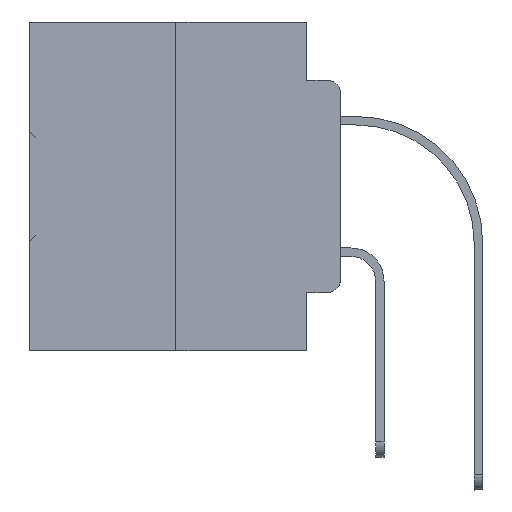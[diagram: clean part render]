
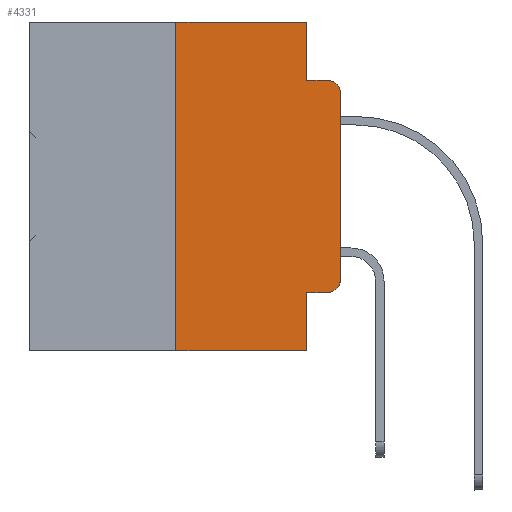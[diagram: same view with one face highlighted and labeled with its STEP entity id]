
A CAD part, left-side view. The second image highlights one B-rep face of the part: STEP entity #4331.
In plain terms, the highlighted planar face has unit normal (-1, 0, 0).
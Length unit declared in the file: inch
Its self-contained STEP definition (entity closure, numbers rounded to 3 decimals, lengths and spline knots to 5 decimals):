
#71 = VERTEX_POINT ( 'NONE', #11386 ) ;
#820 = VECTOR ( 'NONE', #32199, 39.37008 ) ;
#951 = VERTEX_POINT ( 'NONE', #14793 ) ;
#1387 = ORIENTED_EDGE ( 'NONE', *, *, #4646, .T. ) ;
#2530 = CARTESIAN_POINT ( 'NONE',  ( 0., 0.02, -0.1085 ) ) ;
#2739 = CARTESIAN_POINT ( 'NONE',  ( 0., 0.25, 0. ) ) ;
#3098 = VECTOR ( 'NONE', #36138, 39.37008 ) ;
#3519 = AXIS2_PLACEMENT_3D ( 'NONE', #2530, #40285, #39898 ) ;
#3543 = ORIENTED_EDGE ( 'NONE', *, *, #11074, .T. ) ;
#3774 = CARTESIAN_POINT ( 'NONE',  ( 0., 0.25, 0. ) ) ;
#3966 = EDGE_CURVE ( 'NONE', #38152, #21400, #7041, .T. ) ;
#4331 = ADVANCED_FACE ( 'NONE', ( #37162 ), #15233, .F. ) ;
#4646 = EDGE_CURVE ( 'NONE', #7658, #6983, #12684, .T. ) ;
#6547 = ORIENTED_EDGE ( 'NONE', *, *, #21950, .T. ) ;
#6983 = VERTEX_POINT ( 'NONE', #37576 ) ;
#7041 = LINE ( 'NONE', #25828, #21017 ) ;
#7658 = VERTEX_POINT ( 'NONE', #33580 ) ;
#7666 = ORIENTED_EDGE ( 'NONE', *, *, #16347, .F. ) ;
#10382 = ORIENTED_EDGE ( 'NONE', *, *, #17282, .T. ) ;
#11074 = EDGE_CURVE ( 'NONE', #951, #21400, #35186, .T. ) ;
#11386 = CARTESIAN_POINT ( 'NONE',  ( 0., 0.051, 0. ) ) ;
#11757 = CARTESIAN_POINT ( 'NONE',  ( 0., 0.02, -0.0885 ) ) ;
#12130 = VECTOR ( 'NONE', #33326, 39.37008 ) ;
#12591 = VERTEX_POINT ( 'NONE', #33820 ) ;
#12684 = CIRCLE ( 'NONE', #19306, 0.02 ) ;
#13681 = EDGE_CURVE ( 'NONE', #12591, #31669, #24660, .T. ) ;
#13884 = LINE ( 'NONE', #26511, #12130 ) ;
#14793 = CARTESIAN_POINT ( 'NONE',  ( 0., 0., -0.1085 ) ) ;
#14946 = CARTESIAN_POINT ( 'NONE',  ( 0., 0.02, -0.3915 ) ) ;
#15233 = PLANE ( 'NONE',  #28963 ) ;
#16347 = EDGE_CURVE ( 'NONE', #71, #38152, #23553, .T. ) ;
#16421 = CARTESIAN_POINT ( 'NONE',  ( 0., 0.051, -0.5 ) ) ;
#17098 = LINE ( 'NONE', #25800, #820 ) ;
#17282 = EDGE_CURVE ( 'NONE', #6983, #951, #18667, .T. ) ;
#17742 = CARTESIAN_POINT ( 'NONE',  ( 0., 0.051, 0. ) ) ;
#18364 = DIRECTION ( 'NONE',  ( 1., 0., 0. ) ) ;
#18667 = LINE ( 'NONE', #31278, #34180 ) ;
#19306 = AXIS2_PLACEMENT_3D ( 'NONE', #14946, #27579, #31486 ) ;
#19675 = EDGE_LOOP ( 'NONE', ( #10382, #3543, #33241, #7666, #37746, #26493, #24767, #35890, #6547, #1387 ) ) ;
#20393 = CARTESIAN_POINT ( 'NONE',  ( 0., 0.051, 0. ) ) ;
#21017 = VECTOR ( 'NONE', #35334, 39.37008 ) ;
#21400 = VERTEX_POINT ( 'NONE', #11757 ) ;
#21603 = EDGE_CURVE ( 'NONE', #12591, #27173, #17098, .T. ) ;
#21883 = VECTOR ( 'NONE', #37523, 39.37008 ) ;
#21950 = EDGE_CURVE ( 'NONE', #32676, #7658, #37342, .T. ) ;
#23521 = LINE ( 'NONE', #20393, #21883 ) ;
#23553 = LINE ( 'NONE', #17742, #3098 ) ;
#24660 = LINE ( 'NONE', #2739, #35151 ) ;
#24767 = ORIENTED_EDGE ( 'NONE', *, *, #21603, .T. ) ;
#24891 = CARTESIAN_POINT ( 'NONE',  ( 0., 0.051, -0.0885 ) ) ;
#25800 = CARTESIAN_POINT ( 'NONE',  ( 0., 0.473, -0.5 ) ) ;
#25828 = CARTESIAN_POINT ( 'NONE',  ( 0., 0.051, -0.0885 ) ) ;
#26493 = ORIENTED_EDGE ( 'NONE', *, *, #13681, .F. ) ;
#26511 = CARTESIAN_POINT ( 'NONE',  ( 0., 0.473, 0. ) ) ;
#26810 = CARTESIAN_POINT ( 'NONE',  ( 0., 0.051, -0.4115 ) ) ;
#26950 = EDGE_CURVE ( 'NONE', #32676, #27173, #23521, .T. ) ;
#27173 = VERTEX_POINT ( 'NONE', #16421 ) ;
#27264 = CARTESIAN_POINT ( 'NONE',  ( 0., 0.473, 0. ) ) ;
#27377 = DIRECTION ( 'NONE',  ( 0., 0., 1. ) ) ;
#27579 = DIRECTION ( 'NONE',  ( -1., 0., 0. ) ) ;
#28255 = DIRECTION ( 'NONE',  ( 0., -1., 0. ) ) ;
#28668 = EDGE_CURVE ( 'NONE', #31669, #71, #13884, .T. ) ;
#28963 = AXIS2_PLACEMENT_3D ( 'NONE', #27264, #18364, #33637 ) ;
#30565 = VECTOR ( 'NONE', #28255, 39.37008 ) ;
#31278 = CARTESIAN_POINT ( 'NONE',  ( 0., 0., 0. ) ) ;
#31486 = DIRECTION ( 'NONE',  ( 0., 0., -1. ) ) ;
#31669 = VERTEX_POINT ( 'NONE', #3774 ) ;
#31735 = CARTESIAN_POINT ( 'NONE',  ( 0., 0.051, -0.4115 ) ) ;
#32199 = DIRECTION ( 'NONE',  ( 0., -1., 0. ) ) ;
#32676 = VERTEX_POINT ( 'NONE', #26810 ) ;
#33241 = ORIENTED_EDGE ( 'NONE', *, *, #3966, .F. ) ;
#33326 = DIRECTION ( 'NONE',  ( 0., -1., 0. ) ) ;
#33580 = CARTESIAN_POINT ( 'NONE',  ( 0., 0.02, -0.4115 ) ) ;
#33637 = DIRECTION ( 'NONE',  ( 0., 0., -1. ) ) ;
#33820 = CARTESIAN_POINT ( 'NONE',  ( 0., 0.25, -0.5 ) ) ;
#34180 = VECTOR ( 'NONE', #27377, 39.37008 ) ;
#35151 = VECTOR ( 'NONE', #37252, 39.37008 ) ;
#35186 = CIRCLE ( 'NONE', #3519, 0.02 ) ;
#35334 = DIRECTION ( 'NONE',  ( 0., -1., 0. ) ) ;
#35890 = ORIENTED_EDGE ( 'NONE', *, *, #26950, .F. ) ;
#36138 = DIRECTION ( 'NONE',  ( 0., 0., -1. ) ) ;
#37162 = FACE_OUTER_BOUND ( 'NONE', #19675, .T. ) ;
#37252 = DIRECTION ( 'NONE',  ( 0., 0., 1. ) ) ;
#37342 = LINE ( 'NONE', #31735, #30565 ) ;
#37523 = DIRECTION ( 'NONE',  ( 0., 0., -1. ) ) ;
#37576 = CARTESIAN_POINT ( 'NONE',  ( 0., 0., -0.3915 ) ) ;
#37746 = ORIENTED_EDGE ( 'NONE', *, *, #28668, .F. ) ;
#38152 = VERTEX_POINT ( 'NONE', #24891 ) ;
#39898 = DIRECTION ( 'NONE',  ( 0., 0., -1. ) ) ;
#40285 = DIRECTION ( 'NONE',  ( -1., 0., 0. ) ) ;
